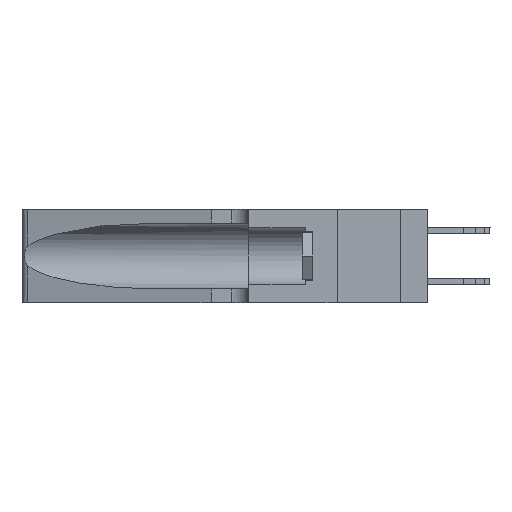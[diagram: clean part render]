
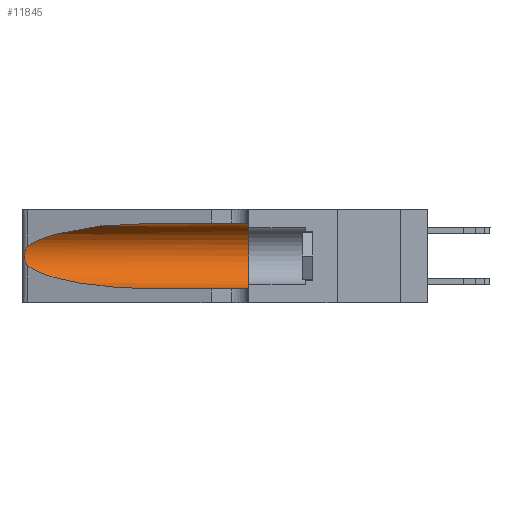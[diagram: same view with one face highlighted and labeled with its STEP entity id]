
A CAD part, left-side view. The second image highlights one B-rep face of the part: STEP entity #11845.
In plain terms, the highlighted cylindrical face has radius 3.308 mm (diameter 6.617 mm), a partial arc.
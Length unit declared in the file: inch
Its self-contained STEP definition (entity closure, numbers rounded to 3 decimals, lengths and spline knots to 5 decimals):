
#873 = CARTESIAN_POINT ( 'NONE',  ( 0.25487, 1.22718, 0.22369 ) ) ;
#1397 = CARTESIAN_POINT ( 'NONE',  ( 0.25487, 1.22718, 0.22369 ) ) ;
#1403 = EDGE_CURVE ( 'NONE', #28599, #9138, #7644, .T. ) ;
#3177 = CARTESIAN_POINT ( 'NONE',  ( 0.25787, 1.23484, 0.2124 ) ) ;
#3295 = CARTESIAN_POINT ( 'NONE',  ( 0.26018, 1.23835, 0.19895 ) ) ;
#3465 = CARTESIAN_POINT ( 'NONE',  ( 0.18966, 0.96281, 0.05475 ) ) ;
#3640 = CARTESIAN_POINT ( 'NONE',  ( 0.25555, 1.22993, 0.14849 ) ) ;
#3686 = ORIENTED_EDGE ( 'NONE', *, *, #8022, .T. ) ;
#4264 = CARTESIAN_POINT ( 'NONE',  ( 0.2373, 1.15595, 0.28018 ) ) ;
#4916 = ORIENTED_EDGE ( 'NONE', *, *, #1403, .F. ) ;
#5309 = AXIS2_PLACEMENT_3D ( 'NONE', #21940, #7777, #19353 ) ;
#6079 = CARTESIAN_POINT ( 'NONE',  ( 0.1305, 0.72297, 0.05475 ) ) ;
#7391 = EDGE_CURVE ( 'NONE', #10275, #19603, #14549, .T. ) ;
#7644 = CIRCLE ( 'NONE', #24609, 0.13025 ) ;
#7777 = DIRECTION ( 'NONE',  ( 0., -1., 0. ) ) ;
#8022 = EDGE_CURVE ( 'NONE', #19603, #21642, #24498, .T. ) ;
#8646 = EDGE_CURVE ( 'NONE', #23495, #10275, #34204, .T. ) ;
#8687 = CYLINDRICAL_SURFACE ( 'NONE', #5309, 0.13025 ) ;
#9036 = CARTESIAN_POINT ( 'NONE',  ( 0.1305, 0.72297, 0.31525 ) ) ;
#9138 = VERTEX_POINT ( 'NONE', #24476 ) ;
#9653 = CARTESIAN_POINT ( 'NONE',  ( 0.1305, 0.72297, 0.31525 ) ) ;
#10275 = VERTEX_POINT ( 'NONE', #873 ) ;
#11440 = ORIENTED_EDGE ( 'NONE', *, *, #8646, .T. ) ;
#11845 = ADVANCED_FACE ( 'NONE', ( #24971 ), #8687, .F. ) ;
#12566 = CARTESIAN_POINT ( 'NONE',  ( 0.25487, 1.22718, 0.14631 ) ) ;
#12608 = EDGE_CURVE ( 'NONE', #23495, #28599, #29404, .T. ) ;
#13830 = CARTESIAN_POINT ( 'NONE',  ( 0.1305, 0.35, 0.31525 ) ) ;
#14461 = CARTESIAN_POINT ( 'NONE',  ( 0.25854, 1.2359, 0.20912 ) ) ;
#14549 = B_SPLINE_CURVE_WITH_KNOTS ( 'NONE', 3,
 ( #28758, #25548, #17542, #3177, #14461, #3295, #28627, #34886, #18035, #23801, #31717, #14829, #3640, #15805 ),
 .UNSPECIFIED., .F., .F.,
 ( 4, 2, 2, 2, 2, 2, 4 ),
 ( 0., 0.00027, 0.00053, 0.00107, 0.0016, 0.00187, 0.00214 ),
 .UNSPECIFIED. ) ;
#14654 = EDGE_CURVE ( 'NONE', #21642, #9138, #22243, .T. ) ;
#14829 = CARTESIAN_POINT ( 'NONE',  ( 0.25639, 1.23186, 0.15144 ) ) ;
#15805 = CARTESIAN_POINT ( 'NONE',  ( 0.25487, 1.22718, 0.14631 ) ) ;
#16401 = DIRECTION ( 'NONE',  ( 0., 0., 1. ) ) ;
#17542 = CARTESIAN_POINT ( 'NONE',  ( 0.25639, 1.23184, 0.21858 ) ) ;
#17970 = EDGE_LOOP ( 'NONE', ( #11440, #18505, #3686, #21547, #4916, #20524 ) ) ;
#18035 = CARTESIAN_POINT ( 'NONE',  ( 0.26017, 1.23833, 0.17102 ) ) ;
#18505 = ORIENTED_EDGE ( 'NONE', *, *, #7391, .T. ) ;
#18519 = CARTESIAN_POINT ( 'NONE',  ( 0.1305, 1.61858, 0.31525 ) ) ;
#19353 = DIRECTION ( 'NONE',  ( 0., 0., -1. ) ) ;
#19372 = DIRECTION ( 'NONE',  ( 0., -1., 0. ) ) ;
#19583 = VECTOR ( 'NONE', #26094, 39.37008 ) ;
#19603 = VERTEX_POINT ( 'NONE', #12566 ) ;
#20410 = CARTESIAN_POINT ( 'NONE',  ( 0.1305, 0.72297, 0.05475 ) ) ;
#20524 = ORIENTED_EDGE ( 'NONE', *, *, #12608, .F. ) ;
#21547 = ORIENTED_EDGE ( 'NONE', *, *, #14654, .T. ) ;
#21642 = VERTEX_POINT ( 'NONE', #6079 ) ;
#21940 = CARTESIAN_POINT ( 'NONE',  ( 0.1305, 1.61858, 0.185 ) ) ;
#22243 = LINE ( 'NONE', #31544, #19583 ) ;
#22893 = CARTESIAN_POINT ( 'NONE',  ( 0.25487, 1.22718, 0.14631 ) ) ;
#23495 = VERTEX_POINT ( 'NONE', #9036 ) ;
#23801 = CARTESIAN_POINT ( 'NONE',  ( 0.25856, 1.23593, 0.16098 ) ) ;
#24476 = CARTESIAN_POINT ( 'NONE',  ( 0.1305, 0.35, 0.05475 ) ) ;
#24498 =( BOUNDED_CURVE ( )  B_SPLINE_CURVE ( 3, ( #22893, #31288, #3465, #20410 ),
 .UNSPECIFIED., .F., .F. ) 
 B_SPLINE_CURVE_WITH_KNOTS ( ( 4, 4 ),
 ( 3.44316, 4.71239 ),
 .UNSPECIFIED. ) 
 CURVE ( )  GEOMETRIC_REPRESENTATION_ITEM ( )  RATIONAL_B_SPLINE_CURVE ( ( 1., 0.87, 0.87, 1. ) ) 
 REPRESENTATION_ITEM ( '' )  );
#24609 = AXIS2_PLACEMENT_3D ( 'NONE', #33295, #33533, #16401 ) ;
#24971 = FACE_OUTER_BOUND ( 'NONE', #17970, .T. ) ;
#25548 = CARTESIAN_POINT ( 'NONE',  ( 0.25555, 1.22994, 0.2215 ) ) ;
#26094 = DIRECTION ( 'NONE',  ( 0., -1., 0. ) ) ;
#28599 = VERTEX_POINT ( 'NONE', #13830 ) ;
#28627 = CARTESIAN_POINT ( 'NONE',  ( 0.26075, 1.23896, 0.19203 ) ) ;
#28758 = CARTESIAN_POINT ( 'NONE',  ( 0.25487, 1.22718, 0.22369 ) ) ;
#29117 = CARTESIAN_POINT ( 'NONE',  ( 0.18966, 0.96281, 0.31525 ) ) ;
#29404 = LINE ( 'NONE', #18519, #31189 ) ;
#31189 = VECTOR ( 'NONE', #19372, 39.37008 ) ;
#31288 = CARTESIAN_POINT ( 'NONE',  ( 0.2373, 1.15595, 0.08982 ) ) ;
#31544 = CARTESIAN_POINT ( 'NONE',  ( 0.1305, 1.61858, 0.05475 ) ) ;
#31717 = CARTESIAN_POINT ( 'NONE',  ( 0.25789, 1.23486, 0.15765 ) ) ;
#33295 = CARTESIAN_POINT ( 'NONE',  ( 0.1305, 0.35, 0.185 ) ) ;
#33533 = DIRECTION ( 'NONE',  ( 0., 1., 0. ) ) ;
#34204 =( BOUNDED_CURVE ( )  B_SPLINE_CURVE ( 3, ( #9653, #29117, #4264, #1397 ),
 .UNSPECIFIED., .F., .F. ) 
 B_SPLINE_CURVE_WITH_KNOTS ( ( 4, 4 ),
 ( 1.5708, 2.84003 ),
 .UNSPECIFIED. ) 
 CURVE ( )  GEOMETRIC_REPRESENTATION_ITEM ( )  RATIONAL_B_SPLINE_CURVE ( ( 1., 0.87, 0.87, 1. ) ) 
 REPRESENTATION_ITEM ( '' )  );
#34886 = CARTESIAN_POINT ( 'NONE',  ( 0.26075, 1.23896, 0.178 ) ) ;
